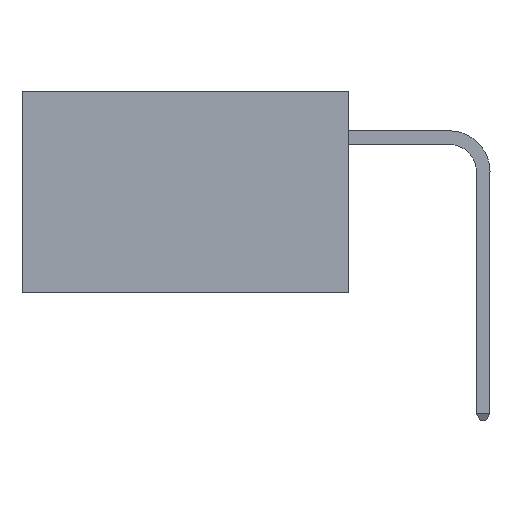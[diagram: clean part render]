
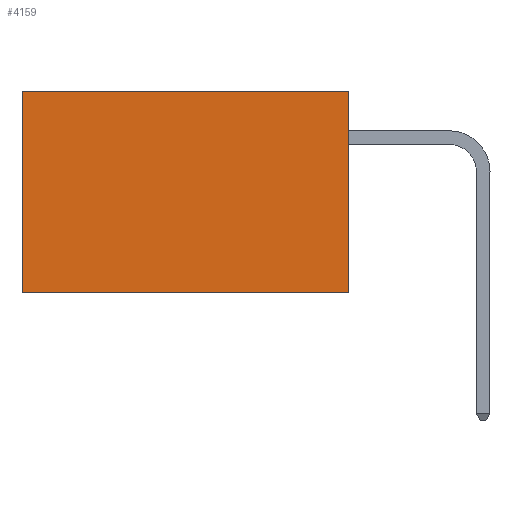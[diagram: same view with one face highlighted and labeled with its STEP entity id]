
A CAD part, left-side view. The second image highlights one B-rep face of the part: STEP entity #4159.
In plain terms, the highlighted planar face has unit normal (-1, 0, 0).
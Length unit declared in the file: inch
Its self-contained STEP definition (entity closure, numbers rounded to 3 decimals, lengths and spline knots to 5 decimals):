
#17 = EDGE_LOOP ( 'NONE', ( #2658, #11516, #11241, #3544 ) ) ;
#72 = CARTESIAN_POINT ( 'NONE',  ( 0.2875, 0.6, 0. ) ) ;
#150 = VERTEX_POINT ( 'NONE', #829 ) ;
#164 = EDGE_CURVE ( 'NONE', #530, #10485, #9471, .T. ) ;
#393 = AXIS2_PLACEMENT_3D ( 'NONE', #8018, #717, #4471 ) ;
#530 = VERTEX_POINT ( 'NONE', #6911 ) ;
#634 = DIRECTION ( 'NONE',  ( 0., 1., 0. ) ) ;
#663 = DIRECTION ( 'NONE',  ( 0., 0., -1. ) ) ;
#717 = DIRECTION ( 'NONE',  ( 1., 0., 0. ) ) ;
#829 = CARTESIAN_POINT ( 'NONE',  ( 0.2875, 0., 0. ) ) ;
#1592 = CARTESIAN_POINT ( 'NONE',  ( 0.2875, 0.6, 0. ) ) ;
#2416 = CARTESIAN_POINT ( 'NONE',  ( 0.2875, 0., 0. ) ) ;
#2658 = ORIENTED_EDGE ( 'NONE', *, *, #9620, .T. ) ;
#2879 = VECTOR ( 'NONE', #663, 39.37008 ) ;
#3187 = LINE ( 'NONE', #1592, #2879 ) ;
#3317 = DIRECTION ( 'NONE',  ( 0., 0., -1. ) ) ;
#3544 = ORIENTED_EDGE ( 'NONE', *, *, #11033, .T. ) ;
#4088 = FACE_OUTER_BOUND ( 'NONE', #17, .T. ) ;
#4159 = ADVANCED_FACE ( 'NONE', ( #4088 ), #8823, .F. ) ;
#4336 = DIRECTION ( 'NONE',  ( 0., 1., 0. ) ) ;
#4471 = DIRECTION ( 'NONE',  ( 0., 0., -1. ) ) ;
#4807 = CARTESIAN_POINT ( 'NONE',  ( 0.2875, 0.6, -0.37 ) ) ;
#5137 = VECTOR ( 'NONE', #3317, 39.37008 ) ;
#6338 = VECTOR ( 'NONE', #4336, 39.37008 ) ;
#6817 = EDGE_CURVE ( 'NONE', #150, #530, #7732, .T. ) ;
#6911 = CARTESIAN_POINT ( 'NONE',  ( 0.2875, 0., -0.37 ) ) ;
#7158 = VERTEX_POINT ( 'NONE', #72 ) ;
#7732 = LINE ( 'NONE', #2416, #5137 ) ;
#8018 = CARTESIAN_POINT ( 'NONE',  ( 0.2875, 0., 0. ) ) ;
#8823 = PLANE ( 'NONE',  #393 ) ;
#9471 = LINE ( 'NONE', #10733, #10921 ) ;
#9620 = EDGE_CURVE ( 'NONE', #7158, #10485, #3187, .T. ) ;
#9656 = CARTESIAN_POINT ( 'NONE',  ( 0.2875, 0., 0. ) ) ;
#10485 = VERTEX_POINT ( 'NONE', #4807 ) ;
#10652 = LINE ( 'NONE', #9656, #6338 ) ;
#10733 = CARTESIAN_POINT ( 'NONE',  ( 0.2875, 0., -0.37 ) ) ;
#10921 = VECTOR ( 'NONE', #634, 39.37008 ) ;
#11033 = EDGE_CURVE ( 'NONE', #150, #7158, #10652, .T. ) ;
#11241 = ORIENTED_EDGE ( 'NONE', *, *, #6817, .F. ) ;
#11516 = ORIENTED_EDGE ( 'NONE', *, *, #164, .F. ) ;
